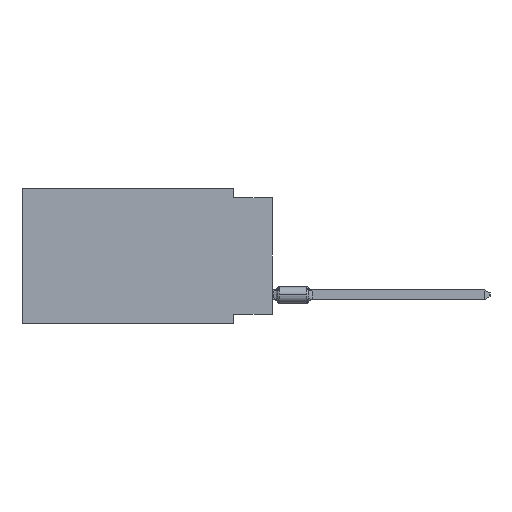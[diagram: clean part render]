
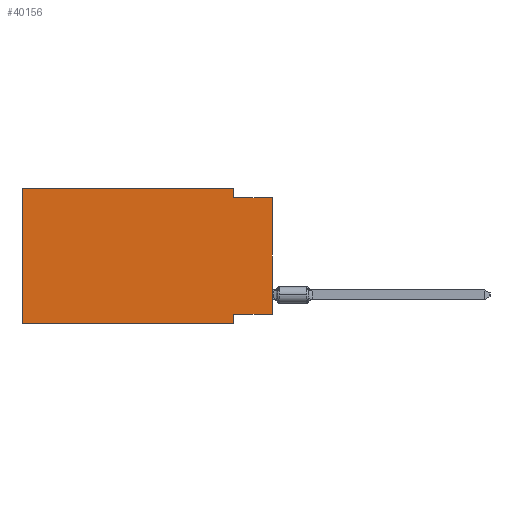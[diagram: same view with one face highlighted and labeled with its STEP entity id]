
A CAD part, left-side view. The second image highlights one B-rep face of the part: STEP entity #40156.
In plain terms, the highlighted planar face has unit normal (-1, 0, 0).
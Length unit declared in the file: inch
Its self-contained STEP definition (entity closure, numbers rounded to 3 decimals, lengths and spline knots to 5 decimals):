
#568 = LINE ( 'NONE', #54955, #35005 ) ;
#1338 = LINE ( 'NONE', #51257, #45738 ) ;
#1571 = DIRECTION ( 'NONE',  ( 0., 0., -1. ) ) ;
#4165 = CARTESIAN_POINT ( 'NONE',  ( 0., 0., -0.325 ) ) ;
#6814 = CARTESIAN_POINT ( 'NONE',  ( 0., 0.645, -0.35 ) ) ;
#6903 = AXIS2_PLACEMENT_3D ( 'NONE', #46732, #24172, #1571 ) ;
#7785 = DIRECTION ( 'NONE',  ( 0., 0., -1. ) ) ;
#8125 = ORIENTED_EDGE ( 'NONE', *, *, #57440, .F. ) ;
#9606 = ORIENTED_EDGE ( 'NONE', *, *, #47858, .T. ) ;
#9968 = DIRECTION ( 'NONE',  ( 0., -1., 0. ) ) ;
#10999 = LINE ( 'NONE', #29140, #34889 ) ;
#12328 = ORIENTED_EDGE ( 'NONE', *, *, #37324, .F. ) ;
#12617 = EDGE_CURVE ( 'NONE', #50152, #36020, #17930, .T. ) ;
#14258 = CARTESIAN_POINT ( 'NONE',  ( 0., 0.1, 0. ) ) ;
#15198 = LINE ( 'NONE', #41326, #45414 ) ;
#17225 = CARTESIAN_POINT ( 'NONE',  ( 0., 0.1, -0.325 ) ) ;
#17519 = DIRECTION ( 'NONE',  ( 0., -1., 0. ) ) ;
#17930 = LINE ( 'NONE', #54755, #27156 ) ;
#21676 = CARTESIAN_POINT ( 'NONE',  ( 0., 0.645, 0. ) ) ;
#23307 = ORIENTED_EDGE ( 'NONE', *, *, #24704, .F. ) ;
#24172 = DIRECTION ( 'NONE',  ( 1., 0., 0. ) ) ;
#24704 = EDGE_CURVE ( 'NONE', #28398, #49271, #15198, .T. ) ;
#26755 = LINE ( 'NONE', #31218, #49521 ) ;
#27156 = VECTOR ( 'NONE', #35477, 39.37008 ) ;
#27613 = CARTESIAN_POINT ( 'NONE',  ( 0., 0.1, -0.025 ) ) ;
#28300 = VERTEX_POINT ( 'NONE', #4165 ) ;
#28398 = VERTEX_POINT ( 'NONE', #14258 ) ;
#28631 = PLANE ( 'NONE',  #6903 ) ;
#29140 = CARTESIAN_POINT ( 'NONE',  ( 0., 0., 0. ) ) ;
#29347 = VECTOR ( 'NONE', #17519, 39.37008 ) ;
#31218 = CARTESIAN_POINT ( 'NONE',  ( 0., 0., -0.325 ) ) ;
#33905 = CARTESIAN_POINT ( 'NONE',  ( 0., 0.1, -0.35 ) ) ;
#33987 = EDGE_CURVE ( 'NONE', #50152, #43778, #568, .T. ) ;
#34889 = VECTOR ( 'NONE', #47533, 39.37008 ) ;
#35005 = VECTOR ( 'NONE', #46024, 39.37008 ) ;
#35477 = DIRECTION ( 'NONE',  ( 0., -1., 0. ) ) ;
#35782 = EDGE_LOOP ( 'NONE', ( #9606, #43242, #23307, #43386, #50208, #50478, #8125, #12328 ) ) ;
#36020 = VERTEX_POINT ( 'NONE', #33905 ) ;
#37324 = EDGE_CURVE ( 'NONE', #28300, #49088, #26755, .T. ) ;
#37536 = FACE_OUTER_BOUND ( 'NONE', #35782, .T. ) ;
#40156 = ADVANCED_FACE ( 'NONE', ( #37536 ), #28631, .F. ) ;
#41326 = CARTESIAN_POINT ( 'NONE',  ( 0., 0.1, 0. ) ) ;
#43242 = ORIENTED_EDGE ( 'NONE', *, *, #53170, .F. ) ;
#43386 = ORIENTED_EDGE ( 'NONE', *, *, #49086, .F. ) ;
#43778 = VERTEX_POINT ( 'NONE', #57006 ) ;
#45414 = VECTOR ( 'NONE', #46672, 39.37008 ) ;
#45424 = LINE ( 'NONE', #21676, #29347 ) ;
#45738 = VECTOR ( 'NONE', #9968, 39.37008 ) ;
#46024 = DIRECTION ( 'NONE',  ( 0., 0., 1. ) ) ;
#46672 = DIRECTION ( 'NONE',  ( 0., 0., -1. ) ) ;
#46732 = CARTESIAN_POINT ( 'NONE',  ( 0., 0.645, 0. ) ) ;
#47479 = CARTESIAN_POINT ( 'NONE',  ( 0., 0., -0.025 ) ) ;
#47533 = DIRECTION ( 'NONE',  ( 0., 0., 1. ) ) ;
#47858 = EDGE_CURVE ( 'NONE', #28300, #49339, #10999, .T. ) ;
#48478 = LINE ( 'NONE', #57709, #52013 ) ;
#49086 = EDGE_CURVE ( 'NONE', #43778, #28398, #45424, .T. ) ;
#49088 = VERTEX_POINT ( 'NONE', #17225 ) ;
#49271 = VERTEX_POINT ( 'NONE', #27613 ) ;
#49339 = VERTEX_POINT ( 'NONE', #47479 ) ;
#49521 = VECTOR ( 'NONE', #49895, 39.37008 ) ;
#49895 = DIRECTION ( 'NONE',  ( 0., 1., 0. ) ) ;
#50152 = VERTEX_POINT ( 'NONE', #6814 ) ;
#50208 = ORIENTED_EDGE ( 'NONE', *, *, #33987, .F. ) ;
#50478 = ORIENTED_EDGE ( 'NONE', *, *, #12617, .T. ) ;
#51257 = CARTESIAN_POINT ( 'NONE',  ( 0., 0., -0.025 ) ) ;
#52013 = VECTOR ( 'NONE', #7785, 39.37008 ) ;
#53170 = EDGE_CURVE ( 'NONE', #49271, #49339, #1338, .T. ) ;
#54755 = CARTESIAN_POINT ( 'NONE',  ( 0., 0.645, -0.35 ) ) ;
#54955 = CARTESIAN_POINT ( 'NONE',  ( 0., 0.645, 0. ) ) ;
#57006 = CARTESIAN_POINT ( 'NONE',  ( 0., 0.645, 0. ) ) ;
#57440 = EDGE_CURVE ( 'NONE', #49088, #36020, #48478, .T. ) ;
#57709 = CARTESIAN_POINT ( 'NONE',  ( 0., 0.1, -0.35 ) ) ;
